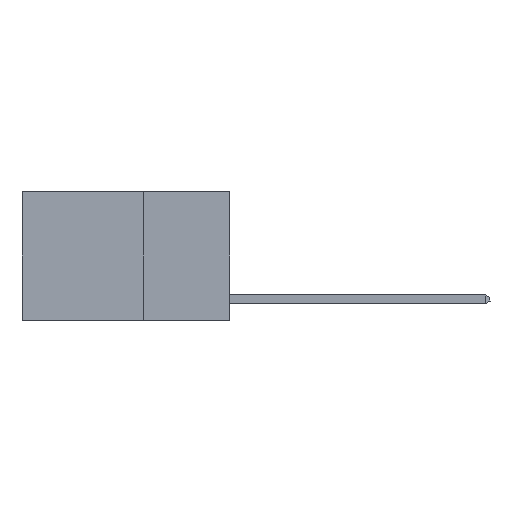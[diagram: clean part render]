
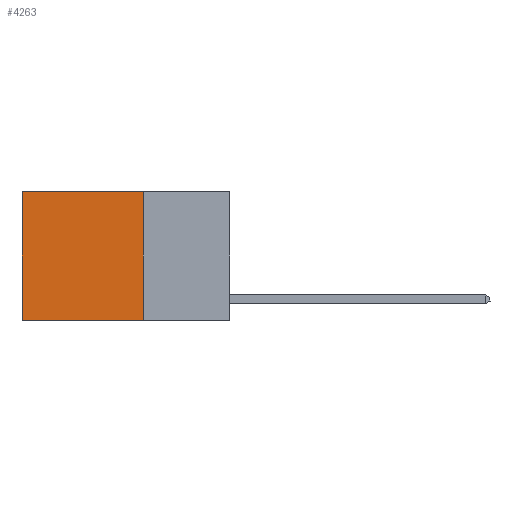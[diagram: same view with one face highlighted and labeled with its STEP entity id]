
A CAD part, left-side view. The second image highlights one B-rep face of the part: STEP entity #4263.
In plain terms, the highlighted planar face has unit normal (-1, 0, 0).
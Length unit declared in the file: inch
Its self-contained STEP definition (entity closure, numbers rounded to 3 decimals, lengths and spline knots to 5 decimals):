
#309 = CARTESIAN_POINT ( 'NONE',  ( 0.2625, 0.25, 0. ) ) ;
#387 = LINE ( 'NONE', #2743, #8375 ) ;
#939 = CARTESIAN_POINT ( 'NONE',  ( 0.2625, 0.6, 0. ) ) ;
#1724 = CARTESIAN_POINT ( 'NONE',  ( 0.2625, 0.6, -0.37 ) ) ;
#2743 = CARTESIAN_POINT ( 'NONE',  ( 0.2625, 0.25, 0. ) ) ;
#2807 = CARTESIAN_POINT ( 'NONE',  ( 0.2625, 0.25, 0. ) ) ;
#2820 = PLANE ( 'NONE',  #7007 ) ;
#2942 = FACE_OUTER_BOUND ( 'NONE', #7748, .T. ) ;
#3988 = EDGE_CURVE ( 'NONE', #11057, #7457, #14610, .T. ) ;
#3993 = DIRECTION ( 'NONE',  ( 0., 0., -1. ) ) ;
#4112 = DIRECTION ( 'NONE',  ( 0., 1., 0. ) ) ;
#4210 = CARTESIAN_POINT ( 'NONE',  ( 0.2625, 0.25, 0. ) ) ;
#4263 = ADVANCED_FACE ( 'NONE', ( #2942 ), #2820, .F. ) ;
#4555 = ORIENTED_EDGE ( 'NONE', *, *, #7357, .F. ) ;
#4996 = EDGE_CURVE ( 'NONE', #11122, #7635, #13109, .T. ) ;
#5492 = VECTOR ( 'NONE', #4112, 39.37008 ) ;
#5811 = EDGE_CURVE ( 'NONE', #7635, #7457, #9517, .T. ) ;
#7007 = AXIS2_PLACEMENT_3D ( 'NONE', #309, #8623, #8714 ) ;
#7357 = EDGE_CURVE ( 'NONE', #11122, #11057, #387, .T. ) ;
#7457 = VERTEX_POINT ( 'NONE', #1724 ) ;
#7628 = CARTESIAN_POINT ( 'NONE',  ( 0.2625, 0.25, -0.37 ) ) ;
#7635 = VERTEX_POINT ( 'NONE', #939 ) ;
#7748 = EDGE_LOOP ( 'NONE', ( #14945, #12181, #4555, #15009 ) ) ;
#8375 = VECTOR ( 'NONE', #3993, 39.37008 ) ;
#8623 = DIRECTION ( 'NONE',  ( 1., 0., 0. ) ) ;
#8714 = DIRECTION ( 'NONE',  ( 0., 0., -1. ) ) ;
#8917 = DIRECTION ( 'NONE',  ( 0., 1., 0. ) ) ;
#9407 = VECTOR ( 'NONE', #8917, 39.37008 ) ;
#9517 = LINE ( 'NONE', #10574, #12157 ) ;
#10574 = CARTESIAN_POINT ( 'NONE',  ( 0.2625, 0.6, 0. ) ) ;
#11057 = VERTEX_POINT ( 'NONE', #7628 ) ;
#11122 = VERTEX_POINT ( 'NONE', #4210 ) ;
#12157 = VECTOR ( 'NONE', #12987, 39.37008 ) ;
#12181 = ORIENTED_EDGE ( 'NONE', *, *, #3988, .F. ) ;
#12987 = DIRECTION ( 'NONE',  ( 0., 0., -1. ) ) ;
#13109 = LINE ( 'NONE', #2807, #5492 ) ;
#14610 = LINE ( 'NONE', #14801, #9407 ) ;
#14801 = CARTESIAN_POINT ( 'NONE',  ( 0.2625, 0.25, -0.37 ) ) ;
#14945 = ORIENTED_EDGE ( 'NONE', *, *, #5811, .T. ) ;
#15009 = ORIENTED_EDGE ( 'NONE', *, *, #4996, .T. ) ;
